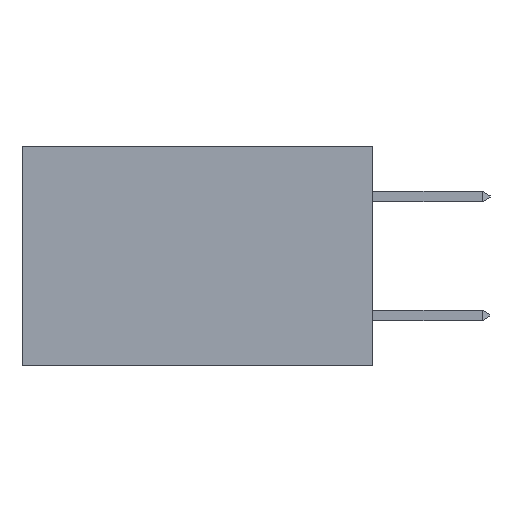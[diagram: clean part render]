
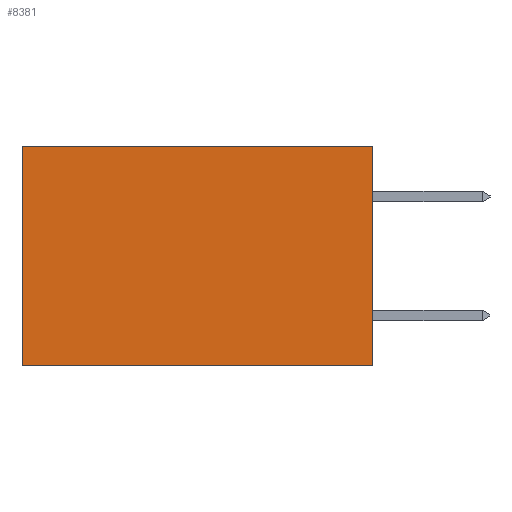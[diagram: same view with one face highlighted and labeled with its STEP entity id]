
A CAD part, left-side view. The second image highlights one B-rep face of the part: STEP entity #8381.
In plain terms, the highlighted planar face has unit normal (-1, 0, 0).
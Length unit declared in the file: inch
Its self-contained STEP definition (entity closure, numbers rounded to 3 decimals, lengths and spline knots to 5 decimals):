
#113 = CARTESIAN_POINT ( 'NONE',  ( 0.277, 0., -0.37 ) ) ;
#167 = DIRECTION ( 'NONE',  ( 1., 0., 0. ) ) ;
#813 = EDGE_CURVE ( 'NONE', #10030, #3660, #7333, .T. ) ;
#1260 = CARTESIAN_POINT ( 'NONE',  ( 0.277, 0.59, -0.37 ) ) ;
#2770 = CARTESIAN_POINT ( 'NONE',  ( 0.277, 0.59, 0. ) ) ;
#2788 = CARTESIAN_POINT ( 'NONE',  ( 0.277, 0.59, -0.37 ) ) ;
#3149 = EDGE_CURVE ( 'NONE', #10030, #11133, #7795, .T. ) ;
#3660 = VERTEX_POINT ( 'NONE', #2770 ) ;
#3888 = DIRECTION ( 'NONE',  ( 0., 0., -1. ) ) ;
#4054 = ORIENTED_EDGE ( 'NONE', *, *, #3149, .F. ) ;
#4095 = LINE ( 'NONE', #2788, #9503 ) ;
#4672 = EDGE_CURVE ( 'NONE', #11133, #5642, #5220, .T. ) ;
#4700 = AXIS2_PLACEMENT_3D ( 'NONE', #13073, #167, #7739 ) ;
#5220 = LINE ( 'NONE', #9255, #13754 ) ;
#5299 = EDGE_LOOP ( 'NONE', ( #9618, #9379, #4054, #9890 ) ) ;
#5565 = CARTESIAN_POINT ( 'NONE',  ( 0.277, 0., -0.37 ) ) ;
#5642 = VERTEX_POINT ( 'NONE', #1260 ) ;
#7118 = VECTOR ( 'NONE', #12245, 39.37008 ) ;
#7333 = LINE ( 'NONE', #7548, #12700 ) ;
#7548 = CARTESIAN_POINT ( 'NONE',  ( 0.277, 0., 0. ) ) ;
#7739 = DIRECTION ( 'NONE',  ( 0., 0., -1. ) ) ;
#7795 = LINE ( 'NONE', #5565, #7118 ) ;
#8002 = DIRECTION ( 'NONE',  ( 0., 1., 0. ) ) ;
#8381 = ADVANCED_FACE ( 'NONE', ( #13200 ), #12009, .F. ) ;
#9255 = CARTESIAN_POINT ( 'NONE',  ( 0.277, 0., -0.37 ) ) ;
#9379 = ORIENTED_EDGE ( 'NONE', *, *, #4672, .F. ) ;
#9503 = VECTOR ( 'NONE', #3888, 39.37008 ) ;
#9618 = ORIENTED_EDGE ( 'NONE', *, *, #11496, .T. ) ;
#9890 = ORIENTED_EDGE ( 'NONE', *, *, #813, .T. ) ;
#10030 = VERTEX_POINT ( 'NONE', #12517 ) ;
#11133 = VERTEX_POINT ( 'NONE', #113 ) ;
#11496 = EDGE_CURVE ( 'NONE', #3660, #5642, #4095, .T. ) ;
#11921 = DIRECTION ( 'NONE',  ( 0., 1., 0. ) ) ;
#12009 = PLANE ( 'NONE',  #4700 ) ;
#12245 = DIRECTION ( 'NONE',  ( 0., 0., -1. ) ) ;
#12517 = CARTESIAN_POINT ( 'NONE',  ( 0.277, 0., 0. ) ) ;
#12700 = VECTOR ( 'NONE', #11921, 39.37008 ) ;
#13073 = CARTESIAN_POINT ( 'NONE',  ( 0.277, 0., -0.37 ) ) ;
#13200 = FACE_OUTER_BOUND ( 'NONE', #5299, .T. ) ;
#13754 = VECTOR ( 'NONE', #8002, 39.37008 ) ;
